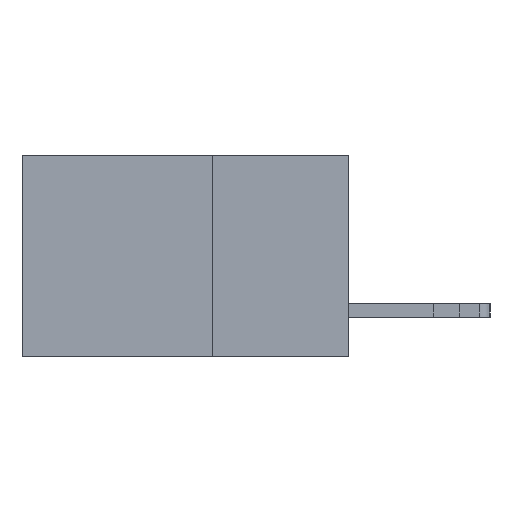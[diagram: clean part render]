
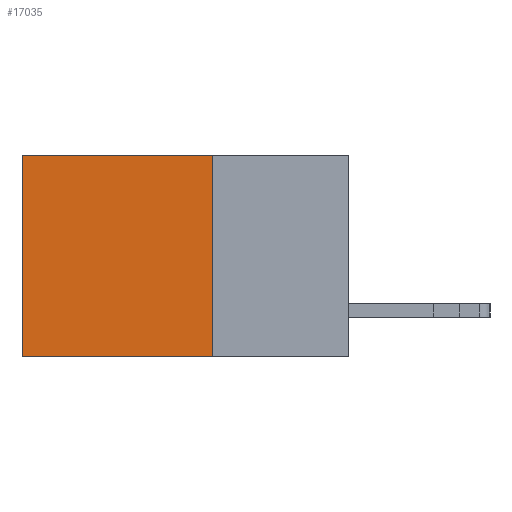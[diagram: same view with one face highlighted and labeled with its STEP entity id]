
A CAD part, left-side view. The second image highlights one B-rep face of the part: STEP entity #17035.
In plain terms, the highlighted planar face has unit normal (-1, 0, 0).
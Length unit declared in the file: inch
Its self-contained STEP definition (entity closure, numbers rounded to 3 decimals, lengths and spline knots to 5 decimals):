
#248 = CARTESIAN_POINT ( 'NONE',  ( 0.298, 0.6, 0. ) ) ;
#1540 = EDGE_CURVE ( 'NONE', #4862, #4532, #3825, .T. ) ;
#1915 = DIRECTION ( 'NONE',  ( 0., 0., -1. ) ) ;
#2035 = FACE_OUTER_BOUND ( 'NONE', #3537, .T. ) ;
#3050 = ORIENTED_EDGE ( 'NONE', *, *, #12260, .T. ) ;
#3537 = EDGE_LOOP ( 'NONE', ( #3050, #13780, #6056, #15296 ) ) ;
#3825 = LINE ( 'NONE', #12343, #20250 ) ;
#4266 = LINE ( 'NONE', #248, #16890 ) ;
#4532 = VERTEX_POINT ( 'NONE', #18466 ) ;
#4862 = VERTEX_POINT ( 'NONE', #17764 ) ;
#5089 = CARTESIAN_POINT ( 'NONE',  ( 0.298, 0.25, 0. ) ) ;
#5657 = CARTESIAN_POINT ( 'NONE',  ( 0.298, 0.6, -0.37 ) ) ;
#6056 = ORIENTED_EDGE ( 'NONE', *, *, #1540, .F. ) ;
#6076 = DIRECTION ( 'NONE',  ( 0., 0., -1. ) ) ;
#6787 = DIRECTION ( 'NONE',  ( 0., 1., 0. ) ) ;
#7365 = DIRECTION ( 'NONE',  ( 1., 0., 0. ) ) ;
#12260 = EDGE_CURVE ( 'NONE', #12486, #13784, #4266, .T. ) ;
#12343 = CARTESIAN_POINT ( 'NONE',  ( 0.298, 0.25, 0. ) ) ;
#12455 = EDGE_CURVE ( 'NONE', #4532, #13784, #13350, .T. ) ;
#12486 = VERTEX_POINT ( 'NONE', #18907 ) ;
#12836 = VECTOR ( 'NONE', #20376, 39.37008 ) ;
#12918 = EDGE_CURVE ( 'NONE', #4862, #12486, #16115, .T. ) ;
#13350 = LINE ( 'NONE', #13956, #12836 ) ;
#13780 = ORIENTED_EDGE ( 'NONE', *, *, #12455, .F. ) ;
#13784 = VERTEX_POINT ( 'NONE', #5657 ) ;
#13901 = CARTESIAN_POINT ( 'NONE',  ( 0.298, 0.25, 0. ) ) ;
#13956 = CARTESIAN_POINT ( 'NONE',  ( 0.298, 0.25, -0.37 ) ) ;
#15296 = ORIENTED_EDGE ( 'NONE', *, *, #12918, .T. ) ;
#16115 = LINE ( 'NONE', #5089, #20894 ) ;
#16890 = VECTOR ( 'NONE', #1915, 39.37008 ) ;
#17035 = ADVANCED_FACE ( 'NONE', ( #2035 ), #17089, .F. ) ;
#17089 = PLANE ( 'NONE',  #17487 ) ;
#17487 = AXIS2_PLACEMENT_3D ( 'NONE', #13901, #7365, #18789 ) ;
#17764 = CARTESIAN_POINT ( 'NONE',  ( 0.298, 0.25, 0. ) ) ;
#18466 = CARTESIAN_POINT ( 'NONE',  ( 0.298, 0.25, -0.37 ) ) ;
#18789 = DIRECTION ( 'NONE',  ( 0., 0., -1. ) ) ;
#18907 = CARTESIAN_POINT ( 'NONE',  ( 0.298, 0.6, 0. ) ) ;
#20250 = VECTOR ( 'NONE', #6076, 39.37008 ) ;
#20376 = DIRECTION ( 'NONE',  ( 0., 1., 0. ) ) ;
#20894 = VECTOR ( 'NONE', #6787, 39.37008 ) ;
